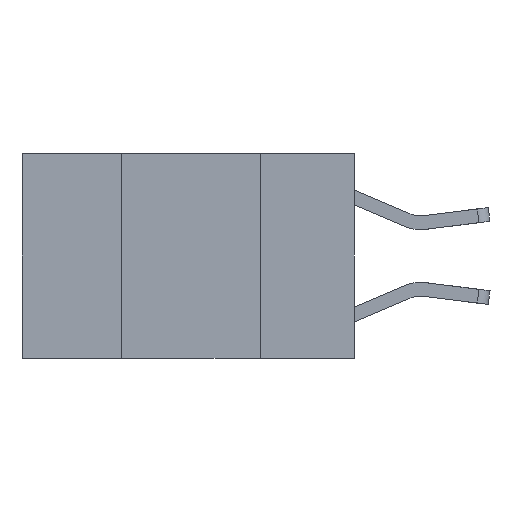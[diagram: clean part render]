
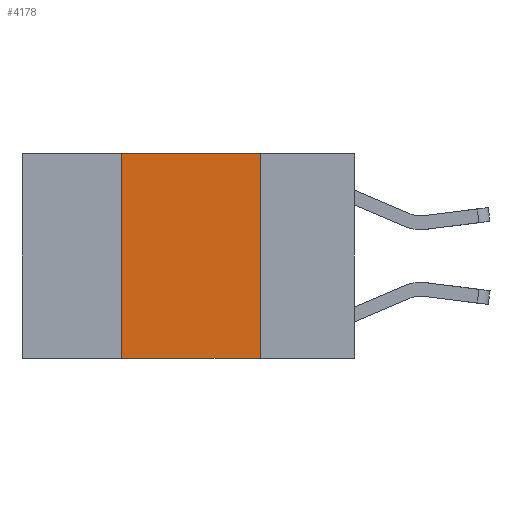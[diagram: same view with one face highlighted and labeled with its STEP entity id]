
A CAD part, left-side view. The second image highlights one B-rep face of the part: STEP entity #4178.
In plain terms, the highlighted planar face has unit normal (-1, 0, 0).
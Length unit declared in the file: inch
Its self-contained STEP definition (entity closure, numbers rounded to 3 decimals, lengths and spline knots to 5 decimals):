
#11 = CARTESIAN_POINT ( 'NONE',  ( 0., 0.17, 0. ) ) ;
#94 = CARTESIAN_POINT ( 'NONE',  ( 0., 0.42, 0. ) ) ;
#584 = CARTESIAN_POINT ( 'NONE',  ( 0., 0.17, 0. ) ) ;
#641 = VECTOR ( 'NONE', #779, 39.37008 ) ;
#689 = EDGE_CURVE ( 'NONE', #3444, #2904, #1233, .T. ) ;
#779 = DIRECTION ( 'NONE',  ( 0., -1., 0. ) ) ;
#821 = VERTEX_POINT ( 'NONE', #94 ) ;
#986 = FACE_OUTER_BOUND ( 'NONE', #6965, .T. ) ;
#1233 = LINE ( 'NONE', #584, #4723 ) ;
#1624 = AXIS2_PLACEMENT_3D ( 'NONE', #7429, #3551, #8083 ) ;
#1767 = DIRECTION ( 'NONE',  ( 0., 0., 1. ) ) ;
#2188 = ORIENTED_EDGE ( 'NONE', *, *, #6204, .F. ) ;
#2904 = VERTEX_POINT ( 'NONE', #5539 ) ;
#2936 = CARTESIAN_POINT ( 'NONE',  ( 0., 0.42, -0.37 ) ) ;
#3014 = VECTOR ( 'NONE', #1767, 39.37008 ) ;
#3107 = DIRECTION ( 'NONE',  ( 0., -1., 0. ) ) ;
#3444 = VERTEX_POINT ( 'NONE', #11 ) ;
#3520 = PLANE ( 'NONE',  #1624 ) ;
#3551 = DIRECTION ( 'NONE',  ( 1., 0., 0. ) ) ;
#3850 = EDGE_CURVE ( 'NONE', #4744, #2904, #4282, .T. ) ;
#4178 = ADVANCED_FACE ( 'NONE', ( #986 ), #3520, .F. ) ;
#4276 = CARTESIAN_POINT ( 'NONE',  ( 0., 0.6, 0. ) ) ;
#4282 = LINE ( 'NONE', #7671, #6052 ) ;
#4369 = LINE ( 'NONE', #4276, #641 ) ;
#4723 = VECTOR ( 'NONE', #5506, 39.37008 ) ;
#4744 = VERTEX_POINT ( 'NONE', #2936 ) ;
#4754 = EDGE_CURVE ( 'NONE', #821, #3444, #4369, .T. ) ;
#4962 = ORIENTED_EDGE ( 'NONE', *, *, #689, .F. ) ;
#5506 = DIRECTION ( 'NONE',  ( 0., 0., -1. ) ) ;
#5539 = CARTESIAN_POINT ( 'NONE',  ( 0., 0.17, -0.37 ) ) ;
#5801 = ORIENTED_EDGE ( 'NONE', *, *, #3850, .T. ) ;
#6052 = VECTOR ( 'NONE', #3107, 39.37008 ) ;
#6204 = EDGE_CURVE ( 'NONE', #4744, #821, #6302, .T. ) ;
#6302 = LINE ( 'NONE', #6482, #3014 ) ;
#6482 = CARTESIAN_POINT ( 'NONE',  ( 0., 0.42, 0. ) ) ;
#6965 = EDGE_LOOP ( 'NONE', ( #4962, #7079, #2188, #5801 ) ) ;
#7079 = ORIENTED_EDGE ( 'NONE', *, *, #4754, .F. ) ;
#7429 = CARTESIAN_POINT ( 'NONE',  ( 0., 0.6, 0. ) ) ;
#7671 = CARTESIAN_POINT ( 'NONE',  ( 0., 0.6, -0.37 ) ) ;
#8083 = DIRECTION ( 'NONE',  ( 0., 0., -1. ) ) ;
